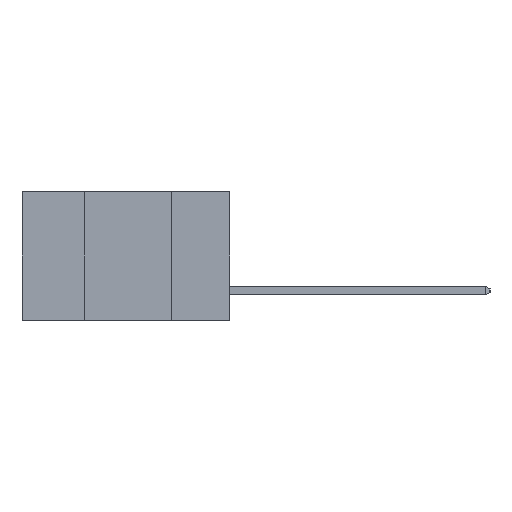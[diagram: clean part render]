
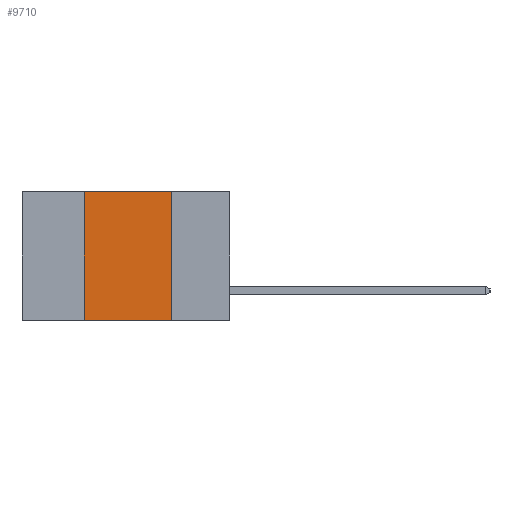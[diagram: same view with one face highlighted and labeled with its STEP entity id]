
A CAD part, left-side view. The second image highlights one B-rep face of the part: STEP entity #9710.
In plain terms, the highlighted planar face has unit normal (-1, 0, 0).
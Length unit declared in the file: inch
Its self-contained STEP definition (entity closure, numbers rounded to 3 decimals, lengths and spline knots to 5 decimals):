
#369 = LINE ( 'NONE', #8315, #8004 ) ;
#513 = EDGE_CURVE ( 'NONE', #1718, #7829, #10918, .T. ) ;
#814 = ORIENTED_EDGE ( 'NONE', *, *, #6116, .F. ) ;
#1718 = VERTEX_POINT ( 'NONE', #8148 ) ;
#2110 = CARTESIAN_POINT ( 'NONE',  ( 0., 0.17, 0. ) ) ;
#2262 = CARTESIAN_POINT ( 'NONE',  ( 0., 0.17, -0.37 ) ) ;
#2276 = DIRECTION ( 'NONE',  ( 0., 0., -1. ) ) ;
#2369 = LINE ( 'NONE', #2262, #4496 ) ;
#2604 = DIRECTION ( 'NONE',  ( 0., 0., 1. ) ) ;
#3014 = DIRECTION ( 'NONE',  ( 0., -1., 0. ) ) ;
#3309 = VECTOR ( 'NONE', #10253, 39.37008 ) ;
#3967 = ORIENTED_EDGE ( 'NONE', *, *, #7960, .F. ) ;
#4173 = PLANE ( 'NONE',  #12422 ) ;
#4496 = VECTOR ( 'NONE', #12929, 39.37008 ) ;
#5253 = EDGE_LOOP ( 'NONE', ( #814, #3967, #11216, #6287 ) ) ;
#5993 = CARTESIAN_POINT ( 'NONE',  ( 0., 0.17, -0.37 ) ) ;
#6116 = EDGE_CURVE ( 'NONE', #8051, #12189, #2369, .T. ) ;
#6199 = FACE_OUTER_BOUND ( 'NONE', #5253, .T. ) ;
#6287 = ORIENTED_EDGE ( 'NONE', *, *, #11428, .T. ) ;
#7229 = CARTESIAN_POINT ( 'NONE',  ( 0., 0.42, 0. ) ) ;
#7596 = DIRECTION ( 'NONE',  ( 1., 0., 0. ) ) ;
#7829 = VERTEX_POINT ( 'NONE', #7229 ) ;
#7960 = EDGE_CURVE ( 'NONE', #7829, #8051, #8812, .T. ) ;
#8004 = VECTOR ( 'NONE', #3014, 39.37008 ) ;
#8051 = VERTEX_POINT ( 'NONE', #2110 ) ;
#8148 = CARTESIAN_POINT ( 'NONE',  ( 0., 0.42, -0.37 ) ) ;
#8315 = CARTESIAN_POINT ( 'NONE',  ( 0., 0.6, -0.37 ) ) ;
#8812 = LINE ( 'NONE', #9286, #3309 ) ;
#9286 = CARTESIAN_POINT ( 'NONE',  ( 0., 0.6, 0. ) ) ;
#9710 = ADVANCED_FACE ( 'NONE', ( #6199 ), #4173, .F. ) ;
#10253 = DIRECTION ( 'NONE',  ( 0., -1., 0. ) ) ;
#10918 = LINE ( 'NONE', #12251, #12281 ) ;
#11216 = ORIENTED_EDGE ( 'NONE', *, *, #513, .F. ) ;
#11428 = EDGE_CURVE ( 'NONE', #1718, #12189, #369, .T. ) ;
#12189 = VERTEX_POINT ( 'NONE', #5993 ) ;
#12251 = CARTESIAN_POINT ( 'NONE',  ( 0., 0.42, -0.37 ) ) ;
#12281 = VECTOR ( 'NONE', #2604, 39.37008 ) ;
#12422 = AXIS2_PLACEMENT_3D ( 'NONE', #13691, #7596, #2276 ) ;
#12929 = DIRECTION ( 'NONE',  ( 0., 0., -1. ) ) ;
#13691 = CARTESIAN_POINT ( 'NONE',  ( 0., 0.6, 0. ) ) ;
